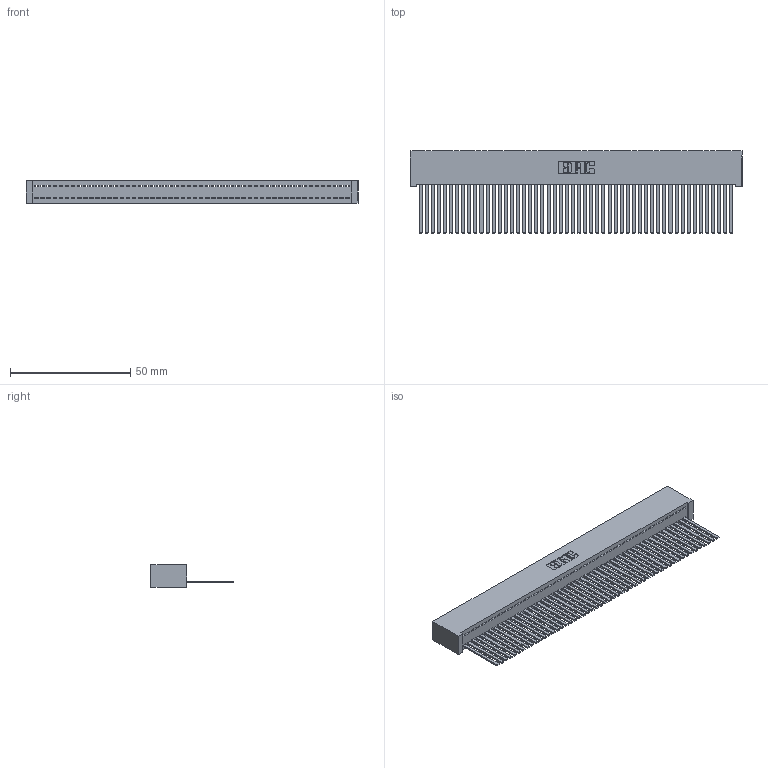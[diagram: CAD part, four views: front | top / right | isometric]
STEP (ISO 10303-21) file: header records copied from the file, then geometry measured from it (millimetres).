
FILE_DESCRIPTION (( 'STEP AP203' ), '1' );
FILE_NAME ('392-052-544-101.STEP', '2018-08-17T05:50:57', ( '' ), ( '' ), 'SwSTEP 2.0', 'SolidWorks 2016', '' );
FILE_SCHEMA (( 'CONFIG_CONTROL_DESIGN' ));
Length unit declared in the file: inch
Products named in the file (3): 392-052-544-101; 342 Part_Lugless; 345-292-001_345-293-144
Assembly tree (53 placements, depth 2):
  392-052-544-101
    342 Part_Lugless
    345-292-001_345-293-144  x52
Bounding box: 138.33 x 34.3 x 9.4 mm (x, y, z)
Volume: 13176.7 mm3; surface area: 21573.3 mm2
Topology: 53 solids, 53 shells, 2806 faces, 8491 edges, 5590 vertices
Faces by surface type: plane 2038, cylinder 768
Entity records: 29903 total; most frequent: CARTESIAN_POINT 5162, ORIENTED_EDGE 5150, DIRECTION 4323, EDGE_CURVE 2575, LINE 2459, VECTOR 2459, VERTEX_POINT 1714, AXIS2_PLACEMENT_3D 932
